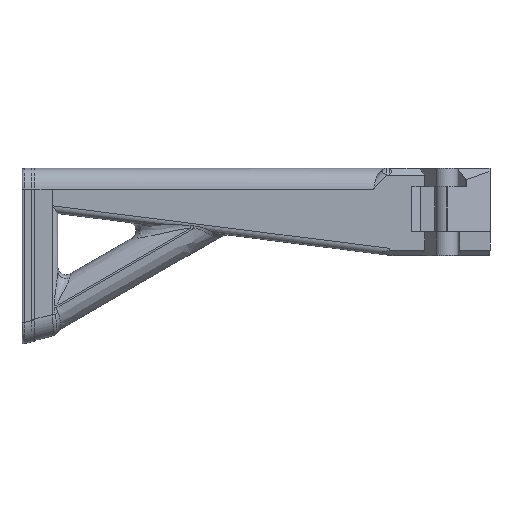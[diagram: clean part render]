
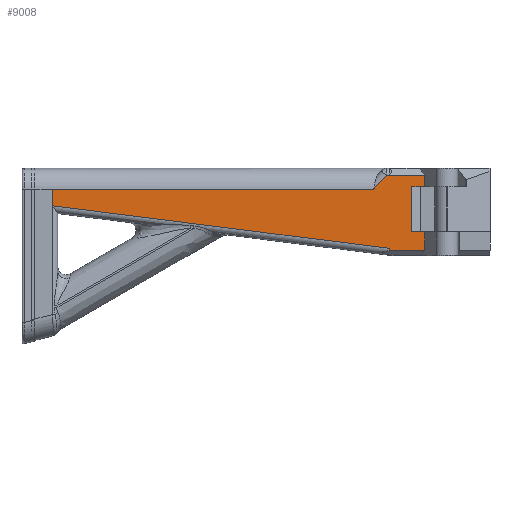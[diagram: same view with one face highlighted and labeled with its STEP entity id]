
A CAD part, top view. The second image highlights one B-rep face of the part: STEP entity #9008.
In plain terms, the highlighted planar face has unit normal (0, 0, 1).
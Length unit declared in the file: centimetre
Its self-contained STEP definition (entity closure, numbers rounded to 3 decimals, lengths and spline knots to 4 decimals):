
#136=B_SPLINE_CURVE_WITH_KNOTS($,3,(#13676,#13677,#13678,#13679,#13680,
#13681,#13682,#13683),.UNSPECIFIED.,.F.,.F.,(4,2,2,4),(0.,
0.0164,0.1084,0.109),.UNSPECIFIED.);
#147=B_SPLINE_CURVE_WITH_KNOTS($,3,(#14263,#14264,#14265,#14266,#14267,
#14268,#14269,#14270,#14271,#14272,#14273,#14274),.UNSPECIFIED.,.F.,.F.,
(4,2,2,2,2,4),(0.0044,0.0052,0.0057,
0.0061,0.0064,0.0065),
 .UNSPECIFIED.);
#974=FACE_OUTER_BOUND($,#1542,.T.);
#1542=EDGE_LOOP($,(#6427,#6428,#6429,#6430,#6431,#6432,#6433,#6434,#6435,
#6436,#6437,#6438,#6439,#6440,#6441));
#2148=LINE($,#13688,#2990);
#2151=LINE($,#13695,#2993);
#2159=LINE($,#13718,#3001);
#2167=LINE($,#13872,#3009);
#2171=LINE($,#13880,#3013);
#2201=LINE($,#13970,#3043);
#2202=LINE($,#13973,#3044);
#2204=LINE($,#13976,#3046);
#2209=LINE($,#13992,#3051);
#2216=LINE($,#14255,#3058);
#2218=LINE($,#14261,#3060);
#2219=LINE($,#14275,#3061);
#2220=LINE($,#14276,#3062);
#2990=VECTOR($,#10737,0.0027);
#2993=VECTOR($,#10742,2.0267);
#3001=VECTOR($,#10764,19.6538);
#3009=VECTOR($,#10786,2.0267);
#3013=VECTOR($,#10792,0.6588);
#3043=VECTOR($,#10874,2.61);
#3044=VECTOR($,#10877,0.7375);
#3046=VECTOR($,#10881,1.075);
#3051=VECTOR($,#10902,0.7375);
#3058=VECTOR($,#10961,1.0702);
#3060=VECTOR($,#10969,18.606);
#3061=VECTOR($,#10970,0.966);
#3062=VECTOR($,#10971,0.1972);
#3809=VERTEX_POINT($,#13673);
#3810=VERTEX_POINT($,#13675);
#3811=VERTEX_POINT($,#13686);
#3814=VERTEX_POINT($,#13693);
#3822=VERTEX_POINT($,#13717);
#3838=VERTEX_POINT($,#13866);
#3840=VERTEX_POINT($,#13871);
#3843=VERTEX_POINT($,#13879);
#3870=VERTEX_POINT($,#13966);
#3871=VERTEX_POINT($,#13968);
#3872=VERTEX_POINT($,#13972);
#3893=VERTEX_POINT($,#14200);
#3895=VERTEX_POINT($,#14206);
#3896=VERTEX_POINT($,#14260);
#3897=VERTEX_POINT($,#14262);
#4698=EDGE_CURVE($,#3809,#3810,#136,.T.);
#4701=EDGE_CURVE($,#3809,#3811,#2148,.T.);
#4704=EDGE_CURVE($,#3814,#3811,#2151,.T.);
#4716=EDGE_CURVE($,#3810,#3822,#2159,.T.);
#4735=EDGE_CURVE($,#3838,#3840,#2167,.T.);
#4739=EDGE_CURVE($,#3840,#3843,#2171,.T.);
#4781=EDGE_CURVE($,#3870,#3871,#2201,.T.);
#4782=EDGE_CURVE($,#3872,#3870,#2202,.T.);
#4784=EDGE_CURVE($,#3872,#3814,#2204,.T.);
#4793=EDGE_CURVE($,#3871,#3843,#2209,.T.);
#4819=EDGE_CURVE($,#3895,#3893,#2216,.T.);
#4822=EDGE_CURVE($,#3896,#3895,#2218,.F.);
#4823=EDGE_CURVE($,#3897,#3896,#147,.T.);
#4824=EDGE_CURVE($,#3822,#3897,#2219,.T.);
#4825=EDGE_CURVE($,#3893,#3838,#2220,.T.);
#6427=ORIENTED_EDGE($,*,*,#4822,.F.);
#6428=ORIENTED_EDGE($,*,*,#4823,.F.);
#6429=ORIENTED_EDGE($,*,*,#4824,.F.);
#6430=ORIENTED_EDGE($,*,*,#4716,.F.);
#6431=ORIENTED_EDGE($,*,*,#4698,.F.);
#6432=ORIENTED_EDGE($,*,*,#4701,.T.);
#6433=ORIENTED_EDGE($,*,*,#4704,.F.);
#6434=ORIENTED_EDGE($,*,*,#4784,.F.);
#6435=ORIENTED_EDGE($,*,*,#4782,.T.);
#6436=ORIENTED_EDGE($,*,*,#4781,.T.);
#6437=ORIENTED_EDGE($,*,*,#4793,.T.);
#6438=ORIENTED_EDGE($,*,*,#4739,.F.);
#6439=ORIENTED_EDGE($,*,*,#4735,.F.);
#6440=ORIENTED_EDGE($,*,*,#4825,.F.);
#6441=ORIENTED_EDGE($,*,*,#4819,.F.);
#8714=PLANE($,#9630);
#9008=ADVANCED_FACE($,(#974),#8714,.F.);
#9630=AXIS2_PLACEMENT_3D($,#14259,#10967,#10968);
#10737=DIRECTION($,(0.,-1.,0.));
#10742=DIRECTION($,(-1.,0.,0.));
#10764=DIRECTION($,(-0.992,0.125,0.));
#10786=DIRECTION($,(1.,0.,0.));
#10792=DIRECTION($,(0.,-1.,0.));
#10874=DIRECTION($,(0.,1.,0.));
#10877=DIRECTION($,(-1.,0.,0.));
#10881=DIRECTION($,(0.,-1.,0.));
#10902=DIRECTION($,(1.,0.,0.));
#10961=DIRECTION($,(0.666,0.746,0.));
#10967=DIRECTION('center_axis',(0.,0.,
-1.));
#10968=DIRECTION('ref_axis',(-1.,0.,0.));
#10969=DIRECTION($,(-1.,0.,0.));
#10970=DIRECTION($,(0.,1.,0.));
#10971=DIRECTION($,(1.,0.,0.));
#13673=CARTESIAN_POINT('',(-25.6136,0.359,11.6297));
#13675=CARTESIAN_POINT('',(-25.6296,0.4742,11.6297));
#13676=CARTESIAN_POINT('Ctrl Pts',(-25.6136,0.359,
11.6297));
#13677=CARTESIAN_POINT('Ctrl Pts',(-25.6136,0.3645,
11.6297));
#13678=CARTESIAN_POINT('Ctrl Pts',(-25.6138,0.37,11.6297));
#13679=CARTESIAN_POINT('Ctrl Pts',(-25.6161,0.4061,
11.6297));
#13680=CARTESIAN_POINT('Ctrl Pts',(-25.6229,0.4404,
11.6297));
#13681=CARTESIAN_POINT('Ctrl Pts',(-25.6295,0.4738,
11.6297));
#13682=CARTESIAN_POINT('Ctrl Pts',(-25.6296,0.474,
11.6297));
#13683=CARTESIAN_POINT('Ctrl Pts',(-25.6296,0.4742,11.6297));
#13686=CARTESIAN_POINT('',(-25.6136,0.3564,11.6297));
#13688=CARTESIAN_POINT($,(-25.6136,1.3961,11.6297));
#13693=CARTESIAN_POINT('',(-23.5869,0.3564,11.6297));
#13695=CARTESIAN_POINT($,(-21.7548,0.3564,11.6297));
#13717=CARTESIAN_POINT('',(-45.1288,2.9342,11.6297));
#13718=CARTESIAN_POINT($,(-26.6097,0.5978,11.6297));
#13866=CARTESIAN_POINT('',(-25.6136,4.7002,11.6297));
#13871=CARTESIAN_POINT('',(-23.5869,4.7002,11.6297));
#13872=CARTESIAN_POINT($,(-21.5906,4.7002,11.6297));
#13879=CARTESIAN_POINT('',(-23.5869,4.0414,11.6297));
#13880=CARTESIAN_POINT($,(-23.5869,2.7314,11.6297));
#13966=CARTESIAN_POINT('',(-24.3244,1.4314,11.6297));
#13968=CARTESIAN_POINT('',(-24.3244,4.0414,11.6297));
#13970=CARTESIAN_POINT($,(-24.3244,2.0489,11.6297));
#13972=CARTESIAN_POINT('',(-23.5869,1.4314,11.6297));
#13973=CARTESIAN_POINT($,(-20.0472,1.4314,11.6297));
#13976=CARTESIAN_POINT($,(-23.5869,0.0564,11.6297));
#13992=CARTESIAN_POINT($,(-20.0279,4.0414,11.6297));
#14200=CARTESIAN_POINT('',(-25.8108,4.7002,11.6297));
#14206=CARTESIAN_POINT('',(-26.5238,3.902,11.6297));
#14255=CARTESIAN_POINT($,(-26.7206,3.6816,11.6297));
#14259=CARTESIAN_POINT('Origin',(-26.5136,2.6,11.6297));
#14260=CARTESIAN_POINT('',(-45.1298,3.902,11.6297));
#14261=CARTESIAN_POINT($,(-46.3298,3.902,11.6297));
#14262=CARTESIAN_POINT('',(-45.1288,3.9002,11.6297));
#14263=CARTESIAN_POINT('Ctrl Pts',(-45.1288,3.9002,11.6297));
#14264=CARTESIAN_POINT('Ctrl Pts',(-45.1288,3.9004,11.6297));
#14265=CARTESIAN_POINT('Ctrl Pts',(-45.1289,3.9008,11.6297));
#14266=CARTESIAN_POINT('Ctrl Pts',(-45.129,3.9012,11.6297));
#14267=CARTESIAN_POINT('Ctrl Pts',(-45.1291,3.9014,11.6297));
#14268=CARTESIAN_POINT('Ctrl Pts',(-45.1292,3.9016,11.6297));
#14269=CARTESIAN_POINT('Ctrl Pts',(-45.1293,3.9017,11.6297));
#14270=CARTESIAN_POINT('Ctrl Pts',(-45.1294,3.9019,11.6297));
#14271=CARTESIAN_POINT('Ctrl Pts',(-45.1295,3.9019,11.6297));
#14272=CARTESIAN_POINT('Ctrl Pts',(-45.1296,3.902,11.6297));
#14273=CARTESIAN_POINT('Ctrl Pts',(-45.1297,3.902,11.6297));
#14274=CARTESIAN_POINT('Ctrl Pts',(-45.1298,3.902,11.6297));
#14275=CARTESIAN_POINT($,(-45.1288,3.7294,11.6297));
#14276=CARTESIAN_POINT($,(-26.5136,4.7002,11.6297));
